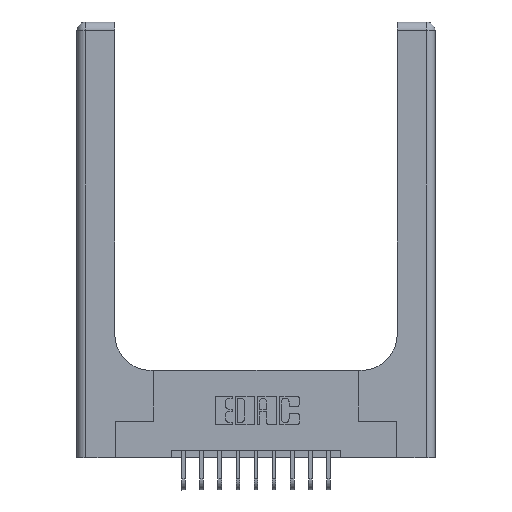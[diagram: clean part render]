
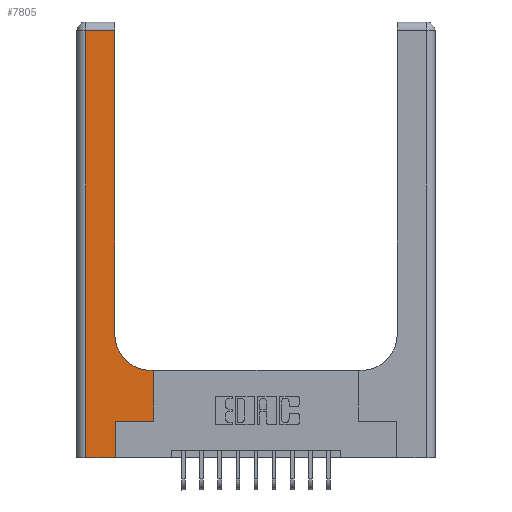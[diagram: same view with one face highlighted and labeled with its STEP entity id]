
A CAD part, top view. The second image highlights one B-rep face of the part: STEP entity #7805.
In plain terms, the highlighted planar face has unit normal (0, 0, 1).
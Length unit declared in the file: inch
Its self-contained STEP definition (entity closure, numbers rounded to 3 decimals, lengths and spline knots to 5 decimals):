
#5 = CARTESIAN_POINT ( 'NONE',  ( 0.06, 0., 0.37 ) ) ;
#149 = EDGE_CURVE ( 'NONE', #15140, #4418, #5757, .T. ) ;
#196 = DIRECTION ( 'NONE',  ( 1., 0., 0. ) ) ;
#234 = VERTEX_POINT ( 'NONE', #13824 ) ;
#612 = VERTEX_POINT ( 'NONE', #11513 ) ;
#849 = ORIENTED_EDGE ( 'NONE', *, *, #4785, .T. ) ;
#922 = EDGE_CURVE ( 'NONE', #234, #16432, #2977, .T. ) ;
#1137 = LINE ( 'NONE', #12853, #15962 ) ;
#1536 = CARTESIAN_POINT ( 'NONE',  ( 0.265, 0., 0.37 ) ) ;
#1750 = ORIENTED_EDGE ( 'NONE', *, *, #6611, .T. ) ;
#2000 = ORIENTED_EDGE ( 'NONE', *, *, #149, .T. ) ;
#2021 = CARTESIAN_POINT ( 'NONE',  ( 0.06, 2.94, 0.37 ) ) ;
#2288 = CARTESIAN_POINT ( 'NONE',  ( 0.528, 0.25, 0.37 ) ) ;
#2535 = VECTOR ( 'NONE', #196, 39.37008 ) ;
#2639 = VERTEX_POINT ( 'NONE', #1536 ) ;
#2877 = CARTESIAN_POINT ( 'NONE',  ( 0.51, 0.85, 0.37 ) ) ;
#2977 = CIRCLE ( 'NONE', #3827, 0.25 ) ;
#3035 = DIRECTION ( 'NONE',  ( -1., 0., 0. ) ) ;
#3388 = CARTESIAN_POINT ( 'NONE',  ( 0.528, 0.6, 0.37 ) ) ;
#3488 = ORIENTED_EDGE ( 'NONE', *, *, #13125, .T. ) ;
#3727 = DIRECTION ( 'NONE',  ( 1., 0., 0. ) ) ;
#3786 = ORIENTED_EDGE ( 'NONE', *, *, #15425, .T. ) ;
#3827 = AXIS2_PLACEMENT_3D ( 'NONE', #2877, #4258, #8147 ) ;
#4113 = VECTOR ( 'NONE', #3727, 39.37008 ) ;
#4258 = DIRECTION ( 'NONE',  ( 0., 0., -1. ) ) ;
#4295 = PLANE ( 'NONE',  #4337 ) ;
#4337 = AXIS2_PLACEMENT_3D ( 'NONE', #9751, #5629, #3035 ) ;
#4418 = VERTEX_POINT ( 'NONE', #3388 ) ;
#4785 = EDGE_CURVE ( 'NONE', #2639, #612, #13135, .T. ) ;
#5004 = ORIENTED_EDGE ( 'NONE', *, *, #922, .T. ) ;
#5260 = VERTEX_POINT ( 'NONE', #5 ) ;
#5376 = LINE ( 'NONE', #11739, #4113 ) ;
#5402 = DIRECTION ( 'NONE',  ( 0., 1., 0. ) ) ;
#5629 = DIRECTION ( 'NONE',  ( 0., 0., -1. ) ) ;
#5757 = LINE ( 'NONE', #12219, #11311 ) ;
#6561 = EDGE_CURVE ( 'NONE', #16955, #5260, #1137, .T. ) ;
#6611 = EDGE_CURVE ( 'NONE', #16432, #16310, #15739, .T. ) ;
#7220 = DIRECTION ( 'NONE',  ( -1., 0., 0. ) ) ;
#7506 = ORIENTED_EDGE ( 'NONE', *, *, #6561, .T. ) ;
#7524 = DIRECTION ( 'NONE',  ( 0., -1., 0. ) ) ;
#7749 = CARTESIAN_POINT ( 'NONE',  ( 0.26, 3., 0.37 ) ) ;
#7805 = ADVANCED_FACE ( 'NONE', ( #9252 ), #4295, .F. ) ;
#8066 = VECTOR ( 'NONE', #14139, 39.37008 ) ;
#8147 = DIRECTION ( 'NONE',  ( 1., 0., 0. ) ) ;
#8517 = CARTESIAN_POINT ( 'NONE',  ( 0., 2.94, 0.37 ) ) ;
#8804 = EDGE_LOOP ( 'NONE', ( #1750, #3786, #7506, #12465, #849, #15331, #2000, #3488, #5004 ) ) ;
#9252 = FACE_OUTER_BOUND ( 'NONE', #8804, .T. ) ;
#9632 = VECTOR ( 'NONE', #7220, 39.37008 ) ;
#9751 = CARTESIAN_POINT ( 'NONE',  ( 0., 3., 0.37 ) ) ;
#10341 = LINE ( 'NONE', #11558, #8066 ) ;
#10625 = CARTESIAN_POINT ( 'NONE',  ( 0.265, 0., 0.37 ) ) ;
#10741 = EDGE_CURVE ( 'NONE', #612, #15140, #5376, .T. ) ;
#10786 = CARTESIAN_POINT ( 'NONE',  ( 0., 0., 0.37 ) ) ;
#11311 = VECTOR ( 'NONE', #5402, 39.37008 ) ;
#11513 = CARTESIAN_POINT ( 'NONE',  ( 0.265, 0.25, 0.37 ) ) ;
#11558 = CARTESIAN_POINT ( 'NONE',  ( 0.26, 0.6, 0.37 ) ) ;
#11739 = CARTESIAN_POINT ( 'NONE',  ( 0.265, 0.25, 0.37 ) ) ;
#12219 = CARTESIAN_POINT ( 'NONE',  ( 0.528, 0.25, 0.37 ) ) ;
#12354 = VECTOR ( 'NONE', #13154, 39.37008 ) ;
#12465 = ORIENTED_EDGE ( 'NONE', *, *, #14053, .T. ) ;
#12853 = CARTESIAN_POINT ( 'NONE',  ( 0.06, 3., 0.37 ) ) ;
#13112 = LINE ( 'NONE', #8517, #9632 ) ;
#13125 = EDGE_CURVE ( 'NONE', #4418, #234, #10341, .T. ) ;
#13135 = LINE ( 'NONE', #10625, #16517 ) ;
#13154 = DIRECTION ( 'NONE',  ( 0., 1., 0. ) ) ;
#13238 = DIRECTION ( 'NONE',  ( 0., 1., 0. ) ) ;
#13824 = CARTESIAN_POINT ( 'NONE',  ( 0.51, 0.6, 0.37 ) ) ;
#14053 = EDGE_CURVE ( 'NONE', #5260, #2639, #16987, .T. ) ;
#14139 = DIRECTION ( 'NONE',  ( -1., 0., 0. ) ) ;
#14787 = CARTESIAN_POINT ( 'NONE',  ( 0.26, 2.94, 0.37 ) ) ;
#15140 = VERTEX_POINT ( 'NONE', #2288 ) ;
#15308 = CARTESIAN_POINT ( 'NONE',  ( 0.26, 0.85, 0.37 ) ) ;
#15331 = ORIENTED_EDGE ( 'NONE', *, *, #10741, .T. ) ;
#15425 = EDGE_CURVE ( 'NONE', #16310, #16955, #13112, .T. ) ;
#15739 = LINE ( 'NONE', #7749, #12354 ) ;
#15962 = VECTOR ( 'NONE', #7524, 39.37008 ) ;
#16310 = VERTEX_POINT ( 'NONE', #14787 ) ;
#16432 = VERTEX_POINT ( 'NONE', #15308 ) ;
#16517 = VECTOR ( 'NONE', #13238, 39.37008 ) ;
#16955 = VERTEX_POINT ( 'NONE', #2021 ) ;
#16987 = LINE ( 'NONE', #10786, #2535 ) ;
